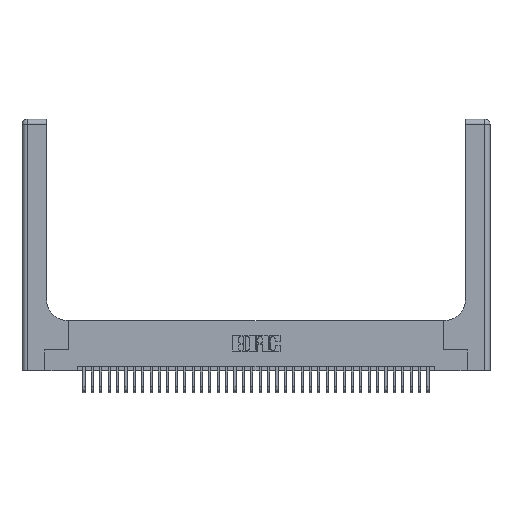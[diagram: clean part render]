
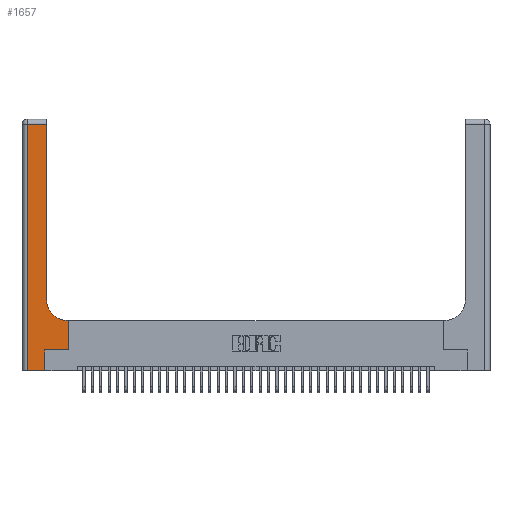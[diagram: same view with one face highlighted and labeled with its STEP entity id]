
A CAD part, top view. The second image highlights one B-rep face of the part: STEP entity #1657.
In plain terms, the highlighted planar face has unit normal (0, 0, 1).
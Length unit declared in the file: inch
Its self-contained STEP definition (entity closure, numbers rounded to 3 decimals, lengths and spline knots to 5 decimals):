
#395 = VERTEX_POINT ( 'NONE', #37668 ) ;
#1224 = EDGE_CURVE ( 'NONE', #17215, #395, #28766, .T. ) ;
#1275 = VECTOR ( 'NONE', #38038, 39.37008 ) ;
#1458 = DIRECTION ( 'NONE',  ( 0., 0., -1. ) ) ;
#1657 = ADVANCED_FACE ( 'NONE', ( #33511 ), #34831, .F. ) ;
#2743 = ORIENTED_EDGE ( 'NONE', *, *, #39413, .T. ) ;
#3339 = EDGE_LOOP ( 'NONE', ( #3965, #38687, #20899, #2743, #23746, #23639, #33819, #26111, #3933 ) ) ;
#3641 = EDGE_CURVE ( 'NONE', #34130, #10638, #21795, .T. ) ;
#3733 = CARTESIAN_POINT ( 'NONE',  ( 0.2915, 0.85, 0.37 ) ) ;
#3745 = VECTOR ( 'NONE', #26691, 39.37008 ) ;
#3770 = VERTEX_POINT ( 'NONE', #35507 ) ;
#3933 = ORIENTED_EDGE ( 'NONE', *, *, #3641, .T. ) ;
#3965 = ORIENTED_EDGE ( 'NONE', *, *, #28775, .T. ) ;
#4153 = CARTESIAN_POINT ( 'NONE',  ( 0., 0., 0.37 ) ) ;
#4791 = CARTESIAN_POINT ( 'NONE',  ( 0.2915, 0.6, 0.37 ) ) ;
#5186 = DIRECTION ( 'NONE',  ( 0., 1., 0. ) ) ;
#5622 = AXIS2_PLACEMENT_3D ( 'NONE', #28950, #16485, #22829 ) ;
#6215 = CARTESIAN_POINT ( 'NONE',  ( 0.5585, 0.25, 0.37 ) ) ;
#6461 = DIRECTION ( 'NONE',  ( 0., 1., 0. ) ) ;
#9633 = EDGE_CURVE ( 'NONE', #22317, #19345, #13681, .T. ) ;
#9832 = LINE ( 'NONE', #35544, #36818 ) ;
#9838 = CARTESIAN_POINT ( 'NONE',  ( 0.06, 2.94, 0.37 ) ) ;
#10638 = VERTEX_POINT ( 'NONE', #3733 ) ;
#13119 = CARTESIAN_POINT ( 'NONE',  ( 0.2915, 3., 0.37 ) ) ;
#13361 = CARTESIAN_POINT ( 'NONE',  ( 0.5415, 0.6, 0.37 ) ) ;
#13681 = LINE ( 'NONE', #22378, #28201 ) ;
#13884 = VECTOR ( 'NONE', #5186, 39.37008 ) ;
#14033 = EDGE_CURVE ( 'NONE', #21708, #22317, #24290, .T. ) ;
#14190 = CARTESIAN_POINT ( 'NONE',  ( 0.5585, 0.25, 0.37 ) ) ;
#14244 = CARTESIAN_POINT ( 'NONE',  ( 0.269, 0.25, 0.37 ) ) ;
#15738 = EDGE_CURVE ( 'NONE', #3770, #34130, #27038, .T. ) ;
#15853 = DIRECTION ( 'NONE',  ( 1., 0., 0. ) ) ;
#16039 = VECTOR ( 'NONE', #6461, 39.37008 ) ;
#16389 = AXIS2_PLACEMENT_3D ( 'NONE', #31387, #1458, #38462 ) ;
#16485 = DIRECTION ( 'NONE',  ( 0., 0., -1. ) ) ;
#17215 = VERTEX_POINT ( 'NONE', #9838 ) ;
#17345 = EDGE_CURVE ( 'NONE', #19345, #3770, #38410, .T. ) ;
#19345 = VERTEX_POINT ( 'NONE', #6215 ) ;
#20213 = VECTOR ( 'NONE', #29282, 39.37008 ) ;
#20899 = ORIENTED_EDGE ( 'NONE', *, *, #1224, .T. ) ;
#21395 = CARTESIAN_POINT ( 'NONE',  ( 0.2915, 2.94, 0.37 ) ) ;
#21708 = VERTEX_POINT ( 'NONE', #23752 ) ;
#21795 = CIRCLE ( 'NONE', #16389, 0.25 ) ;
#22317 = VERTEX_POINT ( 'NONE', #14244 ) ;
#22378 = CARTESIAN_POINT ( 'NONE',  ( 0.269, 0.25, 0.37 ) ) ;
#22829 = DIRECTION ( 'NONE',  ( -1., 0., 0. ) ) ;
#23639 = ORIENTED_EDGE ( 'NONE', *, *, #9633, .T. ) ;
#23746 = ORIENTED_EDGE ( 'NONE', *, *, #14033, .T. ) ;
#23752 = CARTESIAN_POINT ( 'NONE',  ( 0.269, 0., 0.37 ) ) ;
#24290 = LINE ( 'NONE', #35916, #16039 ) ;
#25875 = LINE ( 'NONE', #4153, #1275 ) ;
#26111 = ORIENTED_EDGE ( 'NONE', *, *, #15738, .T. ) ;
#26691 = DIRECTION ( 'NONE',  ( 0., -1., 0. ) ) ;
#27038 = LINE ( 'NONE', #4791, #38480 ) ;
#27109 = CARTESIAN_POINT ( 'NONE',  ( 0.06, 3., 0.37 ) ) ;
#28201 = VECTOR ( 'NONE', #15853, 39.37008 ) ;
#28766 = LINE ( 'NONE', #27109, #3745 ) ;
#28775 = EDGE_CURVE ( 'NONE', #10638, #36871, #32250, .T. ) ;
#28950 = CARTESIAN_POINT ( 'NONE',  ( 0., 3., 0.37 ) ) ;
#29282 = DIRECTION ( 'NONE',  ( 0., 1., 0. ) ) ;
#31387 = CARTESIAN_POINT ( 'NONE',  ( 0.5415, 0.85, 0.37 ) ) ;
#32250 = LINE ( 'NONE', #13119, #20213 ) ;
#32439 = DIRECTION ( 'NONE',  ( -1., 0., 0. ) ) ;
#32479 = DIRECTION ( 'NONE',  ( -1., 0., 0. ) ) ;
#33511 = FACE_OUTER_BOUND ( 'NONE', #3339, .T. ) ;
#33819 = ORIENTED_EDGE ( 'NONE', *, *, #17345, .T. ) ;
#34130 = VERTEX_POINT ( 'NONE', #13361 ) ;
#34831 = PLANE ( 'NONE',  #5622 ) ;
#35507 = CARTESIAN_POINT ( 'NONE',  ( 0.5585, 0.6, 0.37 ) ) ;
#35544 = CARTESIAN_POINT ( 'NONE',  ( 0., 2.94, 0.37 ) ) ;
#35916 = CARTESIAN_POINT ( 'NONE',  ( 0.269, 0., 0.37 ) ) ;
#36818 = VECTOR ( 'NONE', #32439, 39.37008 ) ;
#36871 = VERTEX_POINT ( 'NONE', #21395 ) ;
#37668 = CARTESIAN_POINT ( 'NONE',  ( 0.06, 0., 0.37 ) ) ;
#38038 = DIRECTION ( 'NONE',  ( 1., 0., 0. ) ) ;
#38410 = LINE ( 'NONE', #14190, #13884 ) ;
#38462 = DIRECTION ( 'NONE',  ( 1., 0., 0. ) ) ;
#38480 = VECTOR ( 'NONE', #32479, 39.37008 ) ;
#38687 = ORIENTED_EDGE ( 'NONE', *, *, #38866, .T. ) ;
#38866 = EDGE_CURVE ( 'NONE', #36871, #17215, #9832, .T. ) ;
#39413 = EDGE_CURVE ( 'NONE', #395, #21708, #25875, .T. ) ;
